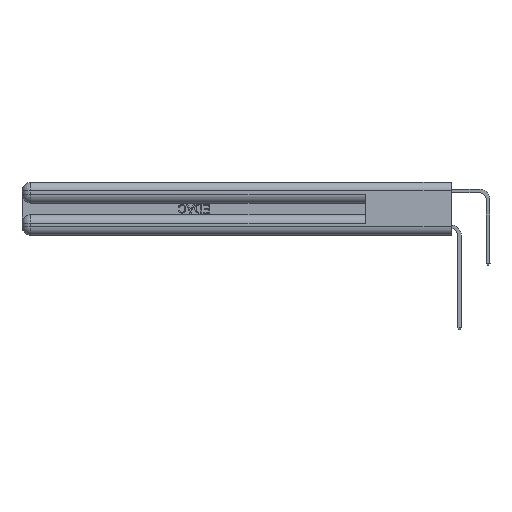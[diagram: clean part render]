
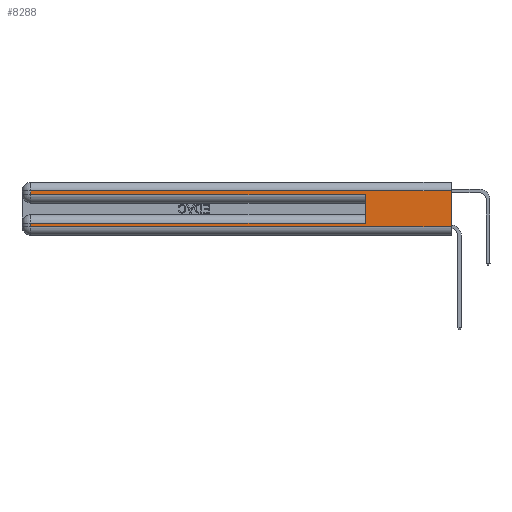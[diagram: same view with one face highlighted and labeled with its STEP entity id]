
A CAD part, left-side view. The second image highlights one B-rep face of the part: STEP entity #8288.
In plain terms, the highlighted planar face has unit normal (-1, 0, 0).
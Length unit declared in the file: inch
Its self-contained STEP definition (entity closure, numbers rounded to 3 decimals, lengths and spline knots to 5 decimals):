
#74 = DIRECTION ( 'NONE',  ( 1., 0., 0. ) ) ;
#532 = CARTESIAN_POINT ( 'NONE',  ( 0., 2.94, 0.37 ) ) ;
#1032 = LINE ( 'NONE', #23815, #24211 ) ;
#1227 = VERTEX_POINT ( 'NONE', #8147 ) ;
#1582 = AXIS2_PLACEMENT_3D ( 'NONE', #20266, #74, #6258 ) ;
#2100 = CARTESIAN_POINT ( 'NONE',  ( 0., 0.6, 0.085 ) ) ;
#2153 = ORIENTED_EDGE ( 'NONE', *, *, #10016, .T. ) ;
#2593 = CARTESIAN_POINT ( 'NONE',  ( 0., 2.94, 0.31 ) ) ;
#2707 = ORIENTED_EDGE ( 'NONE', *, *, #28983, .T. ) ;
#3621 = VERTEX_POINT ( 'NONE', #2593 ) ;
#4374 = VERTEX_POINT ( 'NONE', #10183 ) ;
#5544 = CARTESIAN_POINT ( 'NONE',  ( 0., 0.6, 0.285 ) ) ;
#5887 = PLANE ( 'NONE',  #1582 ) ;
#6258 = DIRECTION ( 'NONE',  ( 0., 0., -1. ) ) ;
#6832 = DIRECTION ( 'NONE',  ( 0., 1., 0. ) ) ;
#6860 = EDGE_CURVE ( 'NONE', #1227, #4374, #8824, .T. ) ;
#7439 = EDGE_CURVE ( 'NONE', #27248, #11353, #34005, .T. ) ;
#8147 = CARTESIAN_POINT ( 'NONE',  ( 0., 2.94, 0.085 ) ) ;
#8288 = ADVANCED_FACE ( 'NONE', ( #9248 ), #5887, .F. ) ;
#8824 = LINE ( 'NONE', #25625, #16578 ) ;
#9248 = FACE_OUTER_BOUND ( 'NONE', #10488, .T. ) ;
#9549 = DIRECTION ( 'NONE',  ( 0., 1., 0. ) ) ;
#9632 = VECTOR ( 'NONE', #31597, 39.37008 ) ;
#10016 = EDGE_CURVE ( 'NONE', #4374, #36396, #32282, .T. ) ;
#10041 = ORIENTED_EDGE ( 'NONE', *, *, #6860, .T. ) ;
#10183 = CARTESIAN_POINT ( 'NONE',  ( 0., 2.94, 0.06 ) ) ;
#10488 = EDGE_LOOP ( 'NONE', ( #29067, #27472, #15479, #2707, #11895, #25877, #10041, #2153 ) ) ;
#11353 = VERTEX_POINT ( 'NONE', #5544 ) ;
#11582 = CARTESIAN_POINT ( 'NONE',  ( 0., 0.6, 0.145 ) ) ;
#11895 = ORIENTED_EDGE ( 'NONE', *, *, #7439, .F. ) ;
#12436 = EDGE_CURVE ( 'NONE', #36867, #3621, #24091, .T. ) ;
#14243 = DIRECTION ( 'NONE',  ( 0., 0., -1. ) ) ;
#14244 = VECTOR ( 'NONE', #15831, 39.37008 ) ;
#15206 = VERTEX_POINT ( 'NONE', #35988 ) ;
#15479 = ORIENTED_EDGE ( 'NONE', *, *, #20622, .T. ) ;
#15831 = DIRECTION ( 'NONE',  ( 0., -1., 0. ) ) ;
#16494 = VECTOR ( 'NONE', #26133, 39.37008 ) ;
#16578 = VECTOR ( 'NONE', #14243, 39.37008 ) ;
#17954 = CARTESIAN_POINT ( 'NONE',  ( 0., 0., 0.37 ) ) ;
#18023 = EDGE_CURVE ( 'NONE', #27248, #1227, #1032, .T. ) ;
#19193 = DIRECTION ( 'NONE',  ( 0., -1., 0. ) ) ;
#20266 = CARTESIAN_POINT ( 'NONE',  ( 0., 0., 0.37 ) ) ;
#20622 = EDGE_CURVE ( 'NONE', #3621, #15206, #20724, .T. ) ;
#20724 = LINE ( 'NONE', #532, #16494 ) ;
#22999 = LINE ( 'NONE', #17954, #9632 ) ;
#23401 = VECTOR ( 'NONE', #19193, 39.37008 ) ;
#23815 = CARTESIAN_POINT ( 'NONE',  ( 0., 0., 0.085 ) ) ;
#24036 = CARTESIAN_POINT ( 'NONE',  ( 0., 0., 0.06 ) ) ;
#24091 = LINE ( 'NONE', #32887, #34747 ) ;
#24211 = VECTOR ( 'NONE', #6832, 39.37008 ) ;
#25625 = CARTESIAN_POINT ( 'NONE',  ( 0., 2.94, 0.37 ) ) ;
#25877 = ORIENTED_EDGE ( 'NONE', *, *, #18023, .T. ) ;
#26133 = DIRECTION ( 'NONE',  ( 0., 0., -1. ) ) ;
#27248 = VERTEX_POINT ( 'NONE', #2100 ) ;
#27276 = EDGE_CURVE ( 'NONE', #36867, #36396, #22999, .T. ) ;
#27472 = ORIENTED_EDGE ( 'NONE', *, *, #12436, .T. ) ;
#27954 = CARTESIAN_POINT ( 'NONE',  ( 0., 0., 0.06 ) ) ;
#28562 = DIRECTION ( 'NONE',  ( 0., 0., 1. ) ) ;
#28983 = EDGE_CURVE ( 'NONE', #15206, #11353, #33398, .T. ) ;
#29067 = ORIENTED_EDGE ( 'NONE', *, *, #27276, .F. ) ;
#30016 = CARTESIAN_POINT ( 'NONE',  ( 0., 0., 0.285 ) ) ;
#31449 = CARTESIAN_POINT ( 'NONE',  ( 0., 0., 0.31 ) ) ;
#31597 = DIRECTION ( 'NONE',  ( 0., 0., -1. ) ) ;
#32282 = LINE ( 'NONE', #24036, #14244 ) ;
#32887 = CARTESIAN_POINT ( 'NONE',  ( 0., 0., 0.31 ) ) ;
#33398 = LINE ( 'NONE', #30016, #23401 ) ;
#33705 = VECTOR ( 'NONE', #28562, 39.37008 ) ;
#34005 = LINE ( 'NONE', #11582, #33705 ) ;
#34747 = VECTOR ( 'NONE', #9549, 39.37008 ) ;
#35988 = CARTESIAN_POINT ( 'NONE',  ( 0., 2.94, 0.285 ) ) ;
#36396 = VERTEX_POINT ( 'NONE', #27954 ) ;
#36867 = VERTEX_POINT ( 'NONE', #31449 ) ;
